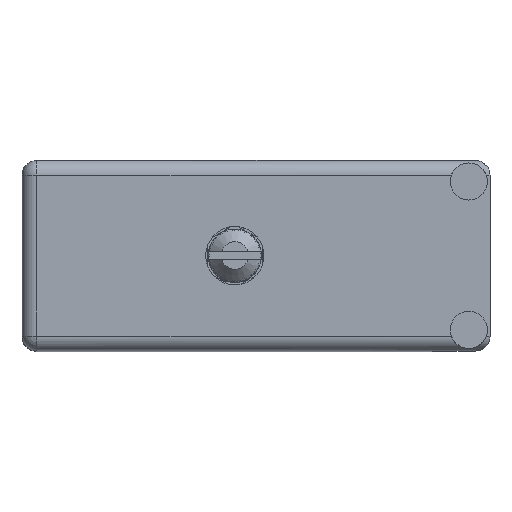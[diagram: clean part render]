
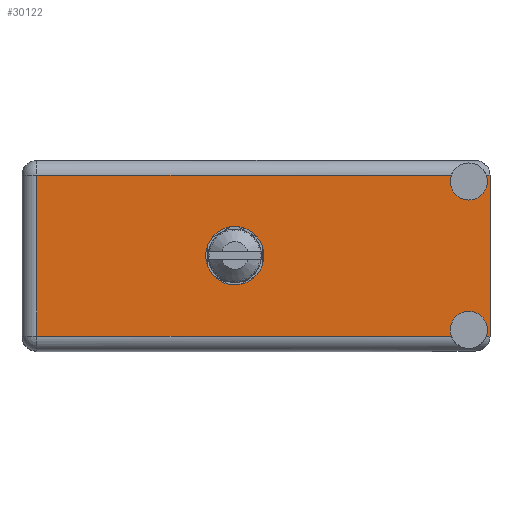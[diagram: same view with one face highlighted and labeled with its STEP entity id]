
A CAD part, top view. The second image highlights one B-rep face of the part: STEP entity #30122.
In plain terms, the highlighted face is planar.
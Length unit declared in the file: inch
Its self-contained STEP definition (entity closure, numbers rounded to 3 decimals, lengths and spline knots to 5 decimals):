
#59 = CARTESIAN_POINT ( 'NONE',  ( 2.108, 1.566, -0.7995 ) ) ;
#187 = VERTEX_POINT ( 'NONE', #7902 ) ;
#1599 = DIRECTION ( 'NONE',  ( -1., 0., 0. ) ) ;
#4068 = EDGE_CURVE ( 'NONE', #13903, #76979, #60130, .T. ) ;
#4088 = AXIS2_PLACEMENT_3D ( 'NONE', #33635, #5541, #112943 ) ;
#4278 = DIRECTION ( 'NONE',  ( 0., 0., 1. ) ) ;
#5541 = DIRECTION ( 'NONE',  ( 0., 1., 0. ) ) ;
#7138 = CARTESIAN_POINT ( 'NONE',  ( 2.208, 1.566, -0.07 ) ) ;
#7902 = CARTESIAN_POINT ( 'NONE',  ( 0.07, 1.566, -0.829 ) ) ;
#10717 = CARTESIAN_POINT ( 'NONE',  ( 1.004, 1.566, -0.4495 ) ) ;
#11762 = EDGE_CURVE ( 'NONE', #76979, #13903, #50848, .T. ) ;
#11972 = CARTESIAN_POINT ( 'NONE',  ( 2.02562, 1.566, -0.07 ) ) ;
#13164 = DIRECTION ( 'NONE',  ( 0., 0., 1. ) ) ;
#13903 = VERTEX_POINT ( 'NONE', #36547 ) ;
#14126 = EDGE_CURVE ( 'NONE', #37869, #56195, #70885, .T. ) ;
#14257 = CARTESIAN_POINT ( 'NONE',  ( 2.108, 1.566, -0.187 ) ) ;
#16053 = DIRECTION ( 'NONE',  ( 1., 0., 0. ) ) ;
#16437 = ORIENTED_EDGE ( 'NONE', *, *, #34009, .F. ) ;
#17271 = ORIENTED_EDGE ( 'NONE', *, *, #11762, .F. ) ;
#18235 = AXIS2_PLACEMENT_3D ( 'NONE', #111375, #40940, #66971 ) ;
#18554 = DIRECTION ( 'NONE',  ( 0., 0., 1. ) ) ;
#20628 = VERTEX_POINT ( 'NONE', #14257 ) ;
#23186 = AXIS2_PLACEMENT_3D ( 'NONE', #59, #63036, #71548 ) ;
#23317 = ORIENTED_EDGE ( 'NONE', *, *, #96122, .F. ) ;
#25024 = ORIENTED_EDGE ( 'NONE', *, *, #67587, .T. ) ;
#26605 = AXIS2_PLACEMENT_3D ( 'NONE', #28708, #71801, #18554 ) ;
#27364 = EDGE_LOOP ( 'NONE', ( #79338, #23317, #36418, #88730, #85118, #25024, #16437, #103561, #110578, #71930 ) ) ;
#28708 = CARTESIAN_POINT ( 'NONE',  ( 2.108, 1.566, -0.0995 ) ) ;
#30046 = EDGE_CURVE ( 'NONE', #94730, #74148, #95991, .T. ) ;
#30122 = ADVANCED_FACE ( 'NONE', ( #74999, #40217 ), #93850, .T. ) ;
#30168 = EDGE_CURVE ( 'NONE', #65032, #56195, #107038, .T. ) ;
#30321 = CARTESIAN_POINT ( 'NONE',  ( 2.208, 1.566, 0. ) ) ;
#30851 = DIRECTION ( 'NONE',  ( -1., 0., 0. ) ) ;
#31131 = VECTOR ( 'NONE', #82651, 39.37008 ) ;
#33635 = CARTESIAN_POINT ( 'NONE',  ( 2.108, 1.566, -0.0995 ) ) ;
#34009 = EDGE_CURVE ( 'NONE', #74148, #103686, #92056, .T. ) ;
#36277 = AXIS2_PLACEMENT_3D ( 'NONE', #49017, #103134, #4278 ) ;
#36418 = ORIENTED_EDGE ( 'NONE', *, *, #37862, .F. ) ;
#36547 = CARTESIAN_POINT ( 'NONE',  ( 1.004, 1.566, -0.312 ) ) ;
#37862 = EDGE_CURVE ( 'NONE', #65032, #20628, #44660, .T. ) ;
#37869 = VERTEX_POINT ( 'NONE', #81944 ) ;
#40217 = FACE_OUTER_BOUND ( 'NONE', #27364, .T. ) ;
#40940 = DIRECTION ( 'NONE',  ( 0., 1., 0. ) ) ;
#40967 = VERTEX_POINT ( 'NONE', #102449 ) ;
#44660 = CIRCLE ( 'NONE', #26605, 0.0875 ) ;
#44663 = EDGE_CURVE ( 'NONE', #40967, #65993, #71613, .T. ) ;
#45842 = AXIS2_PLACEMENT_3D ( 'NONE', #96973, #87922, #51055 ) ;
#49017 = CARTESIAN_POINT ( 'NONE',  ( 1.004, 1.566, -0.4495 ) ) ;
#49297 = CARTESIAN_POINT ( 'NONE',  ( 2.19038, 1.566, -0.07 ) ) ;
#50071 = VECTOR ( 'NONE', #13164, 39.37008 ) ;
#50848 = CIRCLE ( 'NONE', #36277, 0.1375 ) ;
#51055 = DIRECTION ( 'NONE',  ( 0., 0., 1. ) ) ;
#51439 = CARTESIAN_POINT ( 'NONE',  ( 2.208, 1.566, -0.07 ) ) ;
#54046 = VECTOR ( 'NONE', #16053, 39.37008 ) ;
#54859 = CARTESIAN_POINT ( 'NONE',  ( 0., 1.566, -0.829 ) ) ;
#56195 = VERTEX_POINT ( 'NONE', #97878 ) ;
#57000 = CARTESIAN_POINT ( 'NONE',  ( 0.07, 1.566, -0.899 ) ) ;
#60130 = CIRCLE ( 'NONE', #60862, 0.1375 ) ;
#60862 = AXIS2_PLACEMENT_3D ( 'NONE', #10717, #74399, #65093 ) ;
#61126 = LINE ( 'NONE', #110166, #102886 ) ;
#63036 = DIRECTION ( 'NONE',  ( 0., 1., 0. ) ) ;
#65032 = VERTEX_POINT ( 'NONE', #49297 ) ;
#65093 = DIRECTION ( 'NONE',  ( 0., 0., 1. ) ) ;
#65993 = VERTEX_POINT ( 'NONE', #11972 ) ;
#66971 = DIRECTION ( 'NONE',  ( 0., 0., 1. ) ) ;
#67587 = EDGE_CURVE ( 'NONE', #37869, #103686, #106749, .T. ) ;
#68201 = EDGE_LOOP ( 'NONE', ( #111161, #17271 ) ) ;
#68503 = CARTESIAN_POINT ( 'NONE',  ( 1.004, 1.566, -0.587 ) ) ;
#70885 = LINE ( 'NONE', #30321, #50071 ) ;
#71548 = DIRECTION ( 'NONE',  ( 0., 0., 1. ) ) ;
#71613 = LINE ( 'NONE', #7138, #105144 ) ;
#71801 = DIRECTION ( 'NONE',  ( 0., 1., 0. ) ) ;
#71930 = ORIENTED_EDGE ( 'NONE', *, *, #105744, .T. ) ;
#74148 = VERTEX_POINT ( 'NONE', #86812 ) ;
#74399 = DIRECTION ( 'NONE',  ( 0., 1., 0. ) ) ;
#74999 = FACE_BOUND ( 'NONE', #68201, .T. ) ;
#76979 = VERTEX_POINT ( 'NONE', #68503 ) ;
#79338 = ORIENTED_EDGE ( 'NONE', *, *, #44663, .T. ) ;
#81944 = CARTESIAN_POINT ( 'NONE',  ( 2.208, 1.566, -0.829 ) ) ;
#82651 = DIRECTION ( 'NONE',  ( 0., 0., 1. ) ) ;
#85118 = ORIENTED_EDGE ( 'NONE', *, *, #14126, .F. ) ;
#86812 = CARTESIAN_POINT ( 'NONE',  ( 2.108, 1.566, -0.712 ) ) ;
#87922 = DIRECTION ( 'NONE',  ( 0., 1., 0. ) ) ;
#88730 = ORIENTED_EDGE ( 'NONE', *, *, #30168, .T. ) ;
#90937 = CARTESIAN_POINT ( 'NONE',  ( 2.19038, 1.566, -0.829 ) ) ;
#92056 = CIRCLE ( 'NONE', #23186, 0.0875 ) ;
#93850 = PLANE ( 'NONE',  #45842 ) ;
#94730 = VERTEX_POINT ( 'NONE', #94803 ) ;
#94803 = CARTESIAN_POINT ( 'NONE',  ( 2.02562, 1.566, -0.829 ) ) ;
#95991 = CIRCLE ( 'NONE', #18235, 0.0875 ) ;
#96122 = EDGE_CURVE ( 'NONE', #20628, #65993, #101071, .T. ) ;
#96270 = DIRECTION ( 'NONE',  ( 1., 0., 0. ) ) ;
#96973 = CARTESIAN_POINT ( 'NONE',  ( 0., 1.566, -0.899 ) ) ;
#97878 = CARTESIAN_POINT ( 'NONE',  ( 2.208, 1.566, -0.07 ) ) ;
#101071 = CIRCLE ( 'NONE', #4088, 0.0875 ) ;
#102095 = LINE ( 'NONE', #57000, #31131 ) ;
#102449 = CARTESIAN_POINT ( 'NONE',  ( 0.07, 1.566, -0.07 ) ) ;
#102586 = VECTOR ( 'NONE', #1599, 39.37008 ) ;
#102886 = VECTOR ( 'NONE', #30851, 39.37008 ) ;
#103134 = DIRECTION ( 'NONE',  ( 0., 1., 0. ) ) ;
#103561 = ORIENTED_EDGE ( 'NONE', *, *, #30046, .F. ) ;
#103686 = VERTEX_POINT ( 'NONE', #90937 ) ;
#105144 = VECTOR ( 'NONE', #96270, 39.37008 ) ;
#105744 = EDGE_CURVE ( 'NONE', #187, #40967, #102095, .T. ) ;
#106749 = LINE ( 'NONE', #54859, #102586 ) ;
#107038 = LINE ( 'NONE', #51439, #54046 ) ;
#110093 = EDGE_CURVE ( 'NONE', #94730, #187, #61126, .T. ) ;
#110166 = CARTESIAN_POINT ( 'NONE',  ( 0., 1.566, -0.829 ) ) ;
#110578 = ORIENTED_EDGE ( 'NONE', *, *, #110093, .T. ) ;
#111161 = ORIENTED_EDGE ( 'NONE', *, *, #4068, .F. ) ;
#111375 = CARTESIAN_POINT ( 'NONE',  ( 2.108, 1.566, -0.7995 ) ) ;
#112943 = DIRECTION ( 'NONE',  ( 0., 0., 1. ) ) ;
